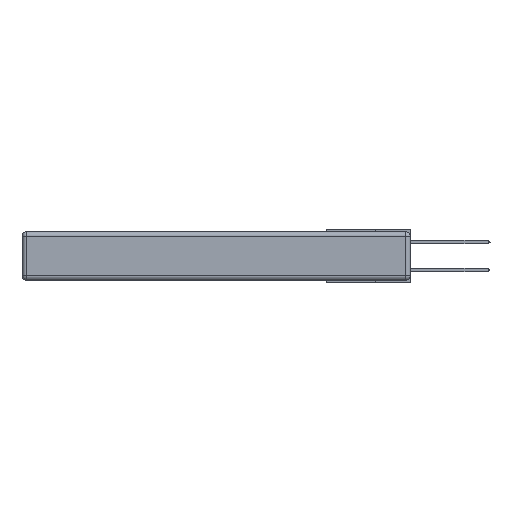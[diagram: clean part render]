
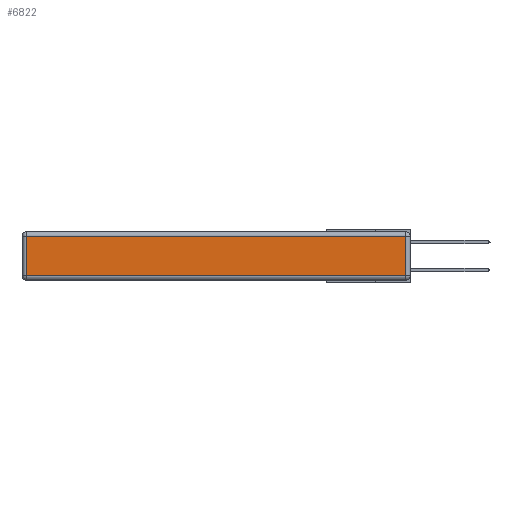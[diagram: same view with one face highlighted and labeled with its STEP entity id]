
A CAD part, left-side view. The second image highlights one B-rep face of the part: STEP entity #6822.
In plain terms, the highlighted planar face has unit normal (-1, 0, 0).
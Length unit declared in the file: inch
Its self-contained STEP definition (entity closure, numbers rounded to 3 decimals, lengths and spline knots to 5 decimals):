
#491 = EDGE_CURVE ( 'NONE', #19022, #24355, #17385, .T. ) ;
#510 = DIRECTION ( 'NONE',  ( 0., 0., -1. ) ) ;
#2435 = CARTESIAN_POINT ( 'NONE',  ( 0., 2.72, -0.313 ) ) ;
#3358 = ORIENTED_EDGE ( 'NONE', *, *, #24634, .T. ) ;
#5492 = VECTOR ( 'NONE', #17472, 39.37008 ) ;
#5749 = CARTESIAN_POINT ( 'NONE',  ( 0., 0.03, -0.343 ) ) ;
#6553 = PLANE ( 'NONE',  #13187 ) ;
#6736 = DIRECTION ( 'NONE',  ( 0., 0., 1. ) ) ;
#6822 = ADVANCED_FACE ( 'NONE', ( #15032 ), #6553, .T. ) ;
#7687 = VECTOR ( 'NONE', #21725, 39.37008 ) ;
#9202 = EDGE_CURVE ( 'NONE', #24355, #23899, #23474, .T. ) ;
#11743 = CARTESIAN_POINT ( 'NONE',  ( 0., 0.03, -0.313 ) ) ;
#11745 = ORIENTED_EDGE ( 'NONE', *, *, #491, .T. ) ;
#13187 = AXIS2_PLACEMENT_3D ( 'NONE', #26912, #26721, #6736 ) ;
#13227 = LINE ( 'NONE', #21866, #5492 ) ;
#13391 = EDGE_CURVE ( 'NONE', #26147, #19022, #18127, .T. ) ;
#13447 = CARTESIAN_POINT ( 'NONE',  ( 0., 2.75, -0.03 ) ) ;
#15032 = FACE_OUTER_BOUND ( 'NONE', #15760, .T. ) ;
#15760 = EDGE_LOOP ( 'NONE', ( #3358, #24632, #11745, #18374 ) ) ;
#17385 = LINE ( 'NONE', #13447, #25032 ) ;
#17472 = DIRECTION ( 'NONE',  ( 0., -1., 0. ) ) ;
#17544 = VECTOR ( 'NONE', #510, 39.37008 ) ;
#18127 = LINE ( 'NONE', #5749, #7687 ) ;
#18374 = ORIENTED_EDGE ( 'NONE', *, *, #9202, .T. ) ;
#19022 = VERTEX_POINT ( 'NONE', #22509 ) ;
#20880 = CARTESIAN_POINT ( 'NONE',  ( 0., 2.72, -0.03 ) ) ;
#21725 = DIRECTION ( 'NONE',  ( 0., 0., 1. ) ) ;
#21866 = CARTESIAN_POINT ( 'NONE',  ( 0., 0., -0.313 ) ) ;
#22509 = CARTESIAN_POINT ( 'NONE',  ( 0., 0.03, -0.03 ) ) ;
#23474 = LINE ( 'NONE', #27401, #17544 ) ;
#23899 = VERTEX_POINT ( 'NONE', #2435 ) ;
#24355 = VERTEX_POINT ( 'NONE', #20880 ) ;
#24606 = DIRECTION ( 'NONE',  ( 0., 1., 0. ) ) ;
#24632 = ORIENTED_EDGE ( 'NONE', *, *, #13391, .T. ) ;
#24634 = EDGE_CURVE ( 'NONE', #23899, #26147, #13227, .T. ) ;
#25032 = VECTOR ( 'NONE', #24606, 39.37008 ) ;
#26147 = VERTEX_POINT ( 'NONE', #11743 ) ;
#26721 = DIRECTION ( 'NONE',  ( -1., 0., 0. ) ) ;
#26912 = CARTESIAN_POINT ( 'NONE',  ( 0., 0., -0.343 ) ) ;
#27401 = CARTESIAN_POINT ( 'NONE',  ( 0., 2.72, -0.343 ) ) ;
